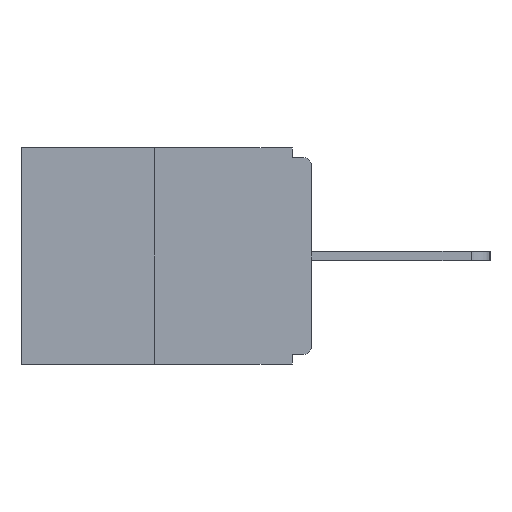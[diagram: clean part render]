
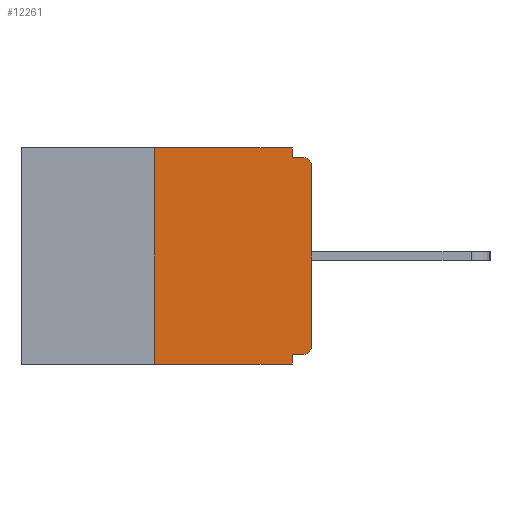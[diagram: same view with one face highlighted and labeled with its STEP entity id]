
A CAD part, left-side view. The second image highlights one B-rep face of the part: STEP entity #12261.
In plain terms, the highlighted planar face has unit normal (-1, 0, 0).
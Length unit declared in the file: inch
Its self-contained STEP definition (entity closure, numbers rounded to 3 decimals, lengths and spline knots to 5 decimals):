
#494 = DIRECTION ( 'NONE',  ( 0., 0., -1. ) ) ;
#594 = CARTESIAN_POINT ( 'NONE',  ( 0., 0.015, -0.015 ) ) ;
#796 = VERTEX_POINT ( 'NONE', #24183 ) ;
#847 = ORIENTED_EDGE ( 'NONE', *, *, #25329, .F. ) ;
#1883 = CIRCLE ( 'NONE', #20130, 0.015 ) ;
#2002 = EDGE_CURVE ( 'NONE', #796, #5411, #8234, .T. ) ;
#2039 = VERTEX_POINT ( 'NONE', #594 ) ;
#2338 = ORIENTED_EDGE ( 'NONE', *, *, #18973, .T. ) ;
#2596 = VERTEX_POINT ( 'NONE', #3853 ) ;
#2928 = CARTESIAN_POINT ( 'NONE',  ( 0., 0.031, -0.015 ) ) ;
#3163 = PLANE ( 'NONE',  #5488 ) ;
#3167 = EDGE_CURVE ( 'NONE', #10221, #2039, #3203, .T. ) ;
#3203 = CIRCLE ( 'NONE', #9820, 0.015 ) ;
#3842 = DIRECTION ( 'NONE',  ( 0., -1., 0. ) ) ;
#3853 = CARTESIAN_POINT ( 'NONE',  ( 0., 0., -0.313 ) ) ;
#3982 = VERTEX_POINT ( 'NONE', #24109 ) ;
#4073 = CARTESIAN_POINT ( 'NONE',  ( 0., 0., -0.03 ) ) ;
#4079 = DIRECTION ( 'NONE',  ( 0., -1., 0. ) ) ;
#4337 = LINE ( 'NONE', #10324, #16987 ) ;
#4772 = CARTESIAN_POINT ( 'NONE',  ( 0., 0.015, -0.328 ) ) ;
#5411 = VERTEX_POINT ( 'NONE', #24222 ) ;
#5430 = VERTEX_POINT ( 'NONE', #2928 ) ;
#5488 = AXIS2_PLACEMENT_3D ( 'NONE', #7285, #7155, #15080 ) ;
#5507 = CARTESIAN_POINT ( 'NONE',  ( 0., 0., -0.015 ) ) ;
#5600 = CARTESIAN_POINT ( 'NONE',  ( 0., 0.031, -0.343 ) ) ;
#5897 = CARTESIAN_POINT ( 'NONE',  ( 0., 0.031, 0. ) ) ;
#6066 = VECTOR ( 'NONE', #13825, 39.37008 ) ;
#7101 = ORIENTED_EDGE ( 'NONE', *, *, #19502, .T. ) ;
#7119 = DIRECTION ( 'NONE',  ( 0., 0., -1. ) ) ;
#7155 = DIRECTION ( 'NONE',  ( 1., 0., 0. ) ) ;
#7285 = CARTESIAN_POINT ( 'NONE',  ( 0., 0.46, 0. ) ) ;
#7296 = LINE ( 'NONE', #5600, #22273 ) ;
#7965 = LINE ( 'NONE', #5507, #14638 ) ;
#8107 = DIRECTION ( 'NONE',  ( 0., 0., 1. ) ) ;
#8234 = LINE ( 'NONE', #9670, #6066 ) ;
#8480 = CARTESIAN_POINT ( 'NONE',  ( 0., 0., -0.328 ) ) ;
#9162 = EDGE_CURVE ( 'NONE', #23593, #23793, #7296, .T. ) ;
#9453 = LINE ( 'NONE', #21276, #9487 ) ;
#9487 = VECTOR ( 'NONE', #3842, 39.37008 ) ;
#9493 = CARTESIAN_POINT ( 'NONE',  ( 0., 0.031, -0.328 ) ) ;
#9670 = CARTESIAN_POINT ( 'NONE',  ( 0., 0.46, 0. ) ) ;
#9820 = AXIS2_PLACEMENT_3D ( 'NONE', #16624, #12867, #7119 ) ;
#10067 = DIRECTION ( 'NONE',  ( 0., 0., -1. ) ) ;
#10221 = VERTEX_POINT ( 'NONE', #4073 ) ;
#10324 = CARTESIAN_POINT ( 'NONE',  ( 0., 0., 0. ) ) ;
#10496 = CARTESIAN_POINT ( 'NONE',  ( 0., 0.015, -0.313 ) ) ;
#12261 = ADVANCED_FACE ( 'NONE', ( #25101 ), #3163, .F. ) ;
#12416 = CARTESIAN_POINT ( 'NONE',  ( 0., 0.25, 0. ) ) ;
#12867 = DIRECTION ( 'NONE',  ( -1., 0., 0. ) ) ;
#13289 = EDGE_LOOP ( 'NONE', ( #23031, #14280, #2338, #21966, #19196, #24035, #7101, #15988, #847, #20294 ) ) ;
#13825 = DIRECTION ( 'NONE',  ( 0., -1., 0. ) ) ;
#14280 = ORIENTED_EDGE ( 'NONE', *, *, #16785, .F. ) ;
#14463 = LINE ( 'NONE', #8480, #23842 ) ;
#14638 = VECTOR ( 'NONE', #4079, 39.37008 ) ;
#15080 = DIRECTION ( 'NONE',  ( 0., 0., -1. ) ) ;
#15414 = EDGE_CURVE ( 'NONE', #17925, #23593, #14463, .T. ) ;
#15988 = ORIENTED_EDGE ( 'NONE', *, *, #3167, .T. ) ;
#16282 = EDGE_CURVE ( 'NONE', #17925, #2596, #1883, .T. ) ;
#16624 = CARTESIAN_POINT ( 'NONE',  ( 0., 0.015, -0.03 ) ) ;
#16785 = EDGE_CURVE ( 'NONE', #3982, #796, #18389, .T. ) ;
#16987 = VECTOR ( 'NONE', #8107, 39.37008 ) ;
#17661 = CARTESIAN_POINT ( 'NONE',  ( 0., 0.031, -0.343 ) ) ;
#17925 = VERTEX_POINT ( 'NONE', #4772 ) ;
#18389 = LINE ( 'NONE', #12416, #20594 ) ;
#18421 = DIRECTION ( 'NONE',  ( -1., 0., 0. ) ) ;
#18973 = EDGE_CURVE ( 'NONE', #3982, #23793, #9453, .T. ) ;
#19196 = ORIENTED_EDGE ( 'NONE', *, *, #15414, .F. ) ;
#19502 = EDGE_CURVE ( 'NONE', #2596, #10221, #4337, .T. ) ;
#19525 = VECTOR ( 'NONE', #10067, 39.37008 ) ;
#20130 = AXIS2_PLACEMENT_3D ( 'NONE', #10496, #18421, #494 ) ;
#20294 = ORIENTED_EDGE ( 'NONE', *, *, #22631, .F. ) ;
#20594 = VECTOR ( 'NONE', #22434, 39.37008 ) ;
#21276 = CARTESIAN_POINT ( 'NONE',  ( 0., 0.46, -0.343 ) ) ;
#21769 = LINE ( 'NONE', #5897, #19525 ) ;
#21966 = ORIENTED_EDGE ( 'NONE', *, *, #9162, .F. ) ;
#22273 = VECTOR ( 'NONE', #24988, 39.37008 ) ;
#22434 = DIRECTION ( 'NONE',  ( 0., 0., 1. ) ) ;
#22538 = DIRECTION ( 'NONE',  ( 0., 1., 0. ) ) ;
#22631 = EDGE_CURVE ( 'NONE', #5411, #5430, #21769, .T. ) ;
#23031 = ORIENTED_EDGE ( 'NONE', *, *, #2002, .F. ) ;
#23593 = VERTEX_POINT ( 'NONE', #9493 ) ;
#23793 = VERTEX_POINT ( 'NONE', #17661 ) ;
#23842 = VECTOR ( 'NONE', #22538, 39.37008 ) ;
#24035 = ORIENTED_EDGE ( 'NONE', *, *, #16282, .T. ) ;
#24109 = CARTESIAN_POINT ( 'NONE',  ( 0., 0.25, -0.343 ) ) ;
#24183 = CARTESIAN_POINT ( 'NONE',  ( 0., 0.25, 0. ) ) ;
#24222 = CARTESIAN_POINT ( 'NONE',  ( 0., 0.031, 0. ) ) ;
#24988 = DIRECTION ( 'NONE',  ( 0., 0., -1. ) ) ;
#25101 = FACE_OUTER_BOUND ( 'NONE', #13289, .T. ) ;
#25329 = EDGE_CURVE ( 'NONE', #5430, #2039, #7965, .T. ) ;
